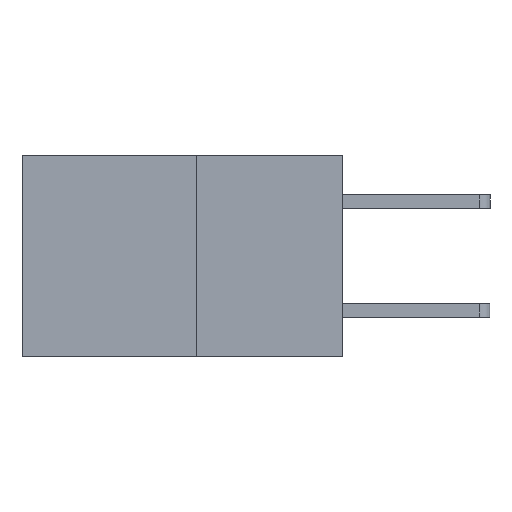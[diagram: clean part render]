
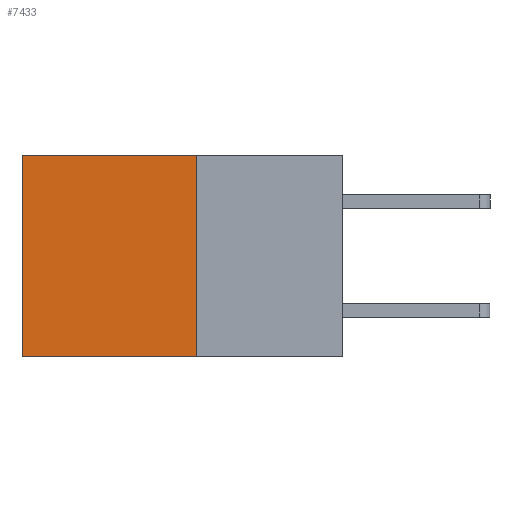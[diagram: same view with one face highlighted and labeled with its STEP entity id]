
A CAD part, left-side view. The second image highlights one B-rep face of the part: STEP entity #7433.
In plain terms, the highlighted planar face has unit normal (-1, 0, 0).
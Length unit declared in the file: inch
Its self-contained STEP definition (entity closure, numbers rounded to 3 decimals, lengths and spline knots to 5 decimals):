
#40 = ORIENTED_EDGE ( 'NONE', *, *, #8142, .F. ) ;
#624 = VERTEX_POINT ( 'NONE', #8365 ) ;
#867 = DIRECTION ( 'NONE',  ( 0., 0., -1. ) ) ;
#980 = VERTEX_POINT ( 'NONE', #3774 ) ;
#1037 = LINE ( 'NONE', #8680, #6597 ) ;
#1232 = CARTESIAN_POINT ( 'NONE',  ( 0.277, 0.59, -0.37 ) ) ;
#1272 = EDGE_CURVE ( 'NONE', #980, #5615, #6300, .T. ) ;
#1599 = ORIENTED_EDGE ( 'NONE', *, *, #6905, .T. ) ;
#1858 = EDGE_LOOP ( 'NONE', ( #1599, #40, #6110, #8475 ) ) ;
#1919 = AXIS2_PLACEMENT_3D ( 'NONE', #7668, #8369, #4028 ) ;
#2640 = FACE_OUTER_BOUND ( 'NONE', #1858, .T. ) ;
#2729 = CARTESIAN_POINT ( 'NONE',  ( 0.277, 0.27, -0.37 ) ) ;
#2743 = VECTOR ( 'NONE', #4116, 39.37008 ) ;
#3112 = VECTOR ( 'NONE', #4852, 39.37008 ) ;
#3323 = LINE ( 'NONE', #1232, #3112 ) ;
#3336 = PLANE ( 'NONE',  #1919 ) ;
#3638 = DIRECTION ( 'NONE',  ( 0., 1., 0. ) ) ;
#3774 = CARTESIAN_POINT ( 'NONE',  ( 0.277, 0.27, 0. ) ) ;
#3871 = EDGE_CURVE ( 'NONE', #980, #624, #1037, .T. ) ;
#4028 = DIRECTION ( 'NONE',  ( 0., 0., -1. ) ) ;
#4116 = DIRECTION ( 'NONE',  ( 0., 1., 0. ) ) ;
#4133 = VECTOR ( 'NONE', #867, 39.37008 ) ;
#4307 = CARTESIAN_POINT ( 'NONE',  ( 0.277, 0.27, -0.37 ) ) ;
#4852 = DIRECTION ( 'NONE',  ( 0., 0., -1. ) ) ;
#5093 = CARTESIAN_POINT ( 'NONE',  ( 0.277, 0.59, -0.37 ) ) ;
#5615 = VERTEX_POINT ( 'NONE', #7046 ) ;
#6110 = ORIENTED_EDGE ( 'NONE', *, *, #1272, .F. ) ;
#6300 = LINE ( 'NONE', #4307, #4133 ) ;
#6597 = VECTOR ( 'NONE', #3638, 39.37008 ) ;
#6905 = EDGE_CURVE ( 'NONE', #624, #7704, #3323, .T. ) ;
#7046 = CARTESIAN_POINT ( 'NONE',  ( 0.277, 0.27, -0.37 ) ) ;
#7433 = ADVANCED_FACE ( 'NONE', ( #2640 ), #3336, .F. ) ;
#7668 = CARTESIAN_POINT ( 'NONE',  ( 0.277, 0.27, -0.37 ) ) ;
#7704 = VERTEX_POINT ( 'NONE', #5093 ) ;
#8032 = LINE ( 'NONE', #2729, #2743 ) ;
#8142 = EDGE_CURVE ( 'NONE', #5615, #7704, #8032, .T. ) ;
#8365 = CARTESIAN_POINT ( 'NONE',  ( 0.277, 0.59, 0. ) ) ;
#8369 = DIRECTION ( 'NONE',  ( 1., 0., 0. ) ) ;
#8475 = ORIENTED_EDGE ( 'NONE', *, *, #3871, .T. ) ;
#8680 = CARTESIAN_POINT ( 'NONE',  ( 0.277, 0.27, 0. ) ) ;
